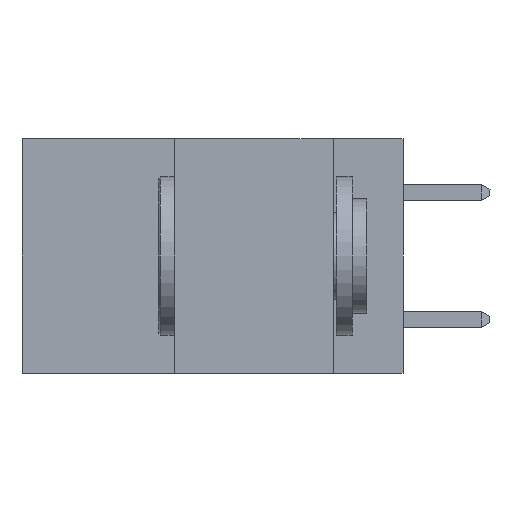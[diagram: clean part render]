
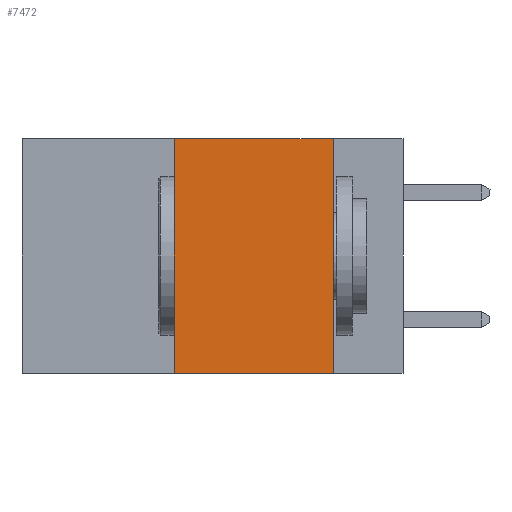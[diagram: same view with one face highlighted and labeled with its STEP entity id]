
A CAD part, left-side view. The second image highlights one B-rep face of the part: STEP entity #7472.
In plain terms, the highlighted planar face has unit normal (-1, 0, 0).
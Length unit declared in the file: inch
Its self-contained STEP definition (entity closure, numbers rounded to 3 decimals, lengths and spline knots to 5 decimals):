
#166 = AXIS2_PLACEMENT_3D ( 'NONE', #172, #3368, #10025 ) ;
#172 = CARTESIAN_POINT ( 'NONE',  ( 0., 0.6, 0. ) ) ;
#340 = VERTEX_POINT ( 'NONE', #12279 ) ;
#780 = CARTESIAN_POINT ( 'NONE',  ( 0., 0.6, 0. ) ) ;
#1176 = DIRECTION ( 'NONE',  ( 0., 0., -1. ) ) ;
#1350 = VECTOR ( 'NONE', #3710, 39.37008 ) ;
#1559 = CARTESIAN_POINT ( 'NONE',  ( 0., 0.11, -0.37 ) ) ;
#1619 = EDGE_CURVE ( 'NONE', #340, #9300, #3774, .T. ) ;
#1713 = EDGE_CURVE ( 'NONE', #11408, #7846, #9847, .T. ) ;
#1797 = CARTESIAN_POINT ( 'NONE',  ( 0., 0.36, 0. ) ) ;
#1955 = EDGE_CURVE ( 'NONE', #11408, #9300, #9089, .T. ) ;
#2347 = PLANE ( 'NONE',  #166 ) ;
#2669 = CARTESIAN_POINT ( 'NONE',  ( 0., 0.11, 0. ) ) ;
#3126 = FACE_OUTER_BOUND ( 'NONE', #4580, .T. ) ;
#3368 = DIRECTION ( 'NONE',  ( 1., 0., 0. ) ) ;
#3707 = CARTESIAN_POINT ( 'NONE',  ( 0., 0.6, -0.37 ) ) ;
#3710 = DIRECTION ( 'NONE',  ( 0., -1., 0. ) ) ;
#3774 = LINE ( 'NONE', #2669, #6091 ) ;
#3908 = DIRECTION ( 'NONE',  ( 0., -1., 0. ) ) ;
#4290 = ORIENTED_EDGE ( 'NONE', *, *, #1619, .F. ) ;
#4547 = ORIENTED_EDGE ( 'NONE', *, *, #1713, .F. ) ;
#4580 = EDGE_LOOP ( 'NONE', ( #4290, #9571, #4547, #7158 ) ) ;
#5481 = VECTOR ( 'NONE', #3908, 39.37008 ) ;
#6091 = VECTOR ( 'NONE', #1176, 39.37008 ) ;
#7158 = ORIENTED_EDGE ( 'NONE', *, *, #1955, .T. ) ;
#7403 = VECTOR ( 'NONE', #7919, 39.37008 ) ;
#7472 = ADVANCED_FACE ( 'NONE', ( #3126 ), #2347, .F. ) ;
#7846 = VERTEX_POINT ( 'NONE', #1797 ) ;
#7919 = DIRECTION ( 'NONE',  ( 0., 0., 1. ) ) ;
#7934 = CARTESIAN_POINT ( 'NONE',  ( 0., 0.36, 0. ) ) ;
#8273 = LINE ( 'NONE', #780, #5481 ) ;
#9089 = LINE ( 'NONE', #3707, #1350 ) ;
#9300 = VERTEX_POINT ( 'NONE', #1559 ) ;
#9571 = ORIENTED_EDGE ( 'NONE', *, *, #11416, .F. ) ;
#9847 = LINE ( 'NONE', #7934, #7403 ) ;
#10025 = DIRECTION ( 'NONE',  ( 0., 0., -1. ) ) ;
#11408 = VERTEX_POINT ( 'NONE', #12104 ) ;
#11416 = EDGE_CURVE ( 'NONE', #7846, #340, #8273, .T. ) ;
#12104 = CARTESIAN_POINT ( 'NONE',  ( 0., 0.36, -0.37 ) ) ;
#12279 = CARTESIAN_POINT ( 'NONE',  ( 0., 0.11, 0. ) ) ;
